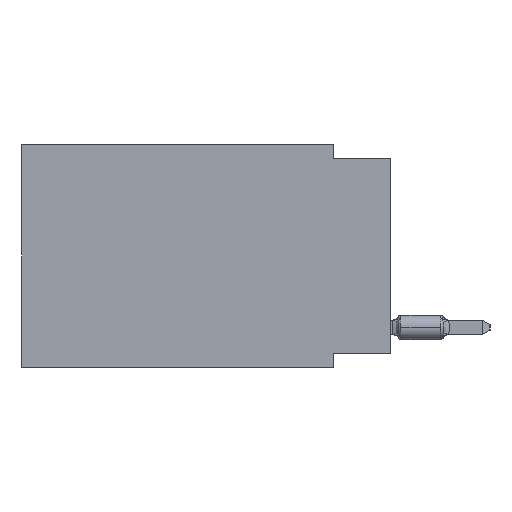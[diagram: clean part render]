
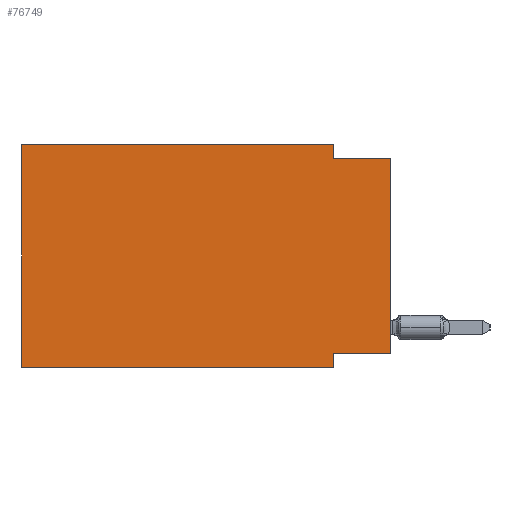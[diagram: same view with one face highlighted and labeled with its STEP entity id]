
A CAD part, left-side view. The second image highlights one B-rep face of the part: STEP entity #76749.
In plain terms, the highlighted planar face has unit normal (-1, 0, 0).
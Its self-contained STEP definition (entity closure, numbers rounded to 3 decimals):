
#1078 = CARTESIAN_POINT ( 'NONE',  ( 0., 0., -9.271 ) ) ;
#1573 = VECTOR ( 'NONE', #29314, 1000. ) ;
#2307 = EDGE_CURVE ( 'NONE', #81047, #10856, #3593, .T. ) ;
#3593 = LINE ( 'NONE', #55426, #55596 ) ;
#5826 = EDGE_CURVE ( 'NONE', #47652, #61496, #57460, .T. ) ;
#7304 = VECTOR ( 'NONE', #48601, 1000. ) ;
#8265 = EDGE_CURVE ( 'NONE', #61496, #81852, #83318, .T. ) ;
#9285 = CARTESIAN_POINT ( 'NONE',  ( 0., 2.54, -9.271 ) ) ;
#9320 = FACE_OUTER_BOUND ( 'NONE', #21078, .T. ) ;
#10399 = CARTESIAN_POINT ( 'NONE',  ( 0., 2.54, -9.906 ) ) ;
#10856 = VERTEX_POINT ( 'NONE', #16833 ) ;
#16367 = DIRECTION ( 'NONE',  ( 0., 0., -1. ) ) ;
#16833 = CARTESIAN_POINT ( 'NONE',  ( 0., 2.54, -9.906 ) ) ;
#18100 = ORIENTED_EDGE ( 'NONE', *, *, #40704, .F. ) ;
#21078 = EDGE_LOOP ( 'NONE', ( #23453, #83665, #46682, #51522, #18100, #27784, #24920, #65943 ) ) ;
#22477 = DIRECTION ( 'NONE',  ( 0., 0., -1. ) ) ;
#23117 = VERTEX_POINT ( 'NONE', #81016 ) ;
#23349 = CARTESIAN_POINT ( 'NONE',  ( 0., 0., 0. ) ) ;
#23400 = CARTESIAN_POINT ( 'NONE',  ( 0., 16.383, 0. ) ) ;
#23453 = ORIENTED_EDGE ( 'NONE', *, *, #25530, .T. ) ;
#24920 = ORIENTED_EDGE ( 'NONE', *, *, #61089, .F. ) ;
#25530 = EDGE_CURVE ( 'NONE', #64119, #81852, #73940, .T. ) ;
#27784 = ORIENTED_EDGE ( 'NONE', *, *, #2307, .T. ) ;
#28859 = CARTESIAN_POINT ( 'NONE',  ( 0., 16.383, 0. ) ) ;
#29314 = DIRECTION ( 'NONE',  ( 0., 0., 1. ) ) ;
#29662 = VECTOR ( 'NONE', #16367, 1000. ) ;
#30366 = LINE ( 'NONE', #10399, #29662 ) ;
#33137 = VECTOR ( 'NONE', #68941, 1000. ) ;
#35249 = PLANE ( 'NONE',  #65870 ) ;
#35443 = CARTESIAN_POINT ( 'NONE',  ( 0., 0., -9.271 ) ) ;
#36220 = EDGE_CURVE ( 'NONE', #64119, #68903, #67724, .T. ) ;
#37059 = CARTESIAN_POINT ( 'NONE',  ( 0., 16.383, -9.906 ) ) ;
#37674 = VECTOR ( 'NONE', #42556, 1000. ) ;
#40704 = EDGE_CURVE ( 'NONE', #81047, #23117, #56981, .T. ) ;
#42556 = DIRECTION ( 'NONE',  ( 0., 0., 1. ) ) ;
#43032 = CARTESIAN_POINT ( 'NONE',  ( 0., 2.54, 0. ) ) ;
#46682 = ORIENTED_EDGE ( 'NONE', *, *, #5826, .F. ) ;
#47134 = CARTESIAN_POINT ( 'NONE',  ( 0., 2.54, 0. ) ) ;
#47652 = VERTEX_POINT ( 'NONE', #47134 ) ;
#48601 = DIRECTION ( 'NONE',  ( 0., 1., 0. ) ) ;
#49036 = DIRECTION ( 'NONE',  ( 0., -1., 0. ) ) ;
#51522 = ORIENTED_EDGE ( 'NONE', *, *, #60721, .F. ) ;
#54775 = DIRECTION ( 'NONE',  ( 1., 0., 0. ) ) ;
#55426 = CARTESIAN_POINT ( 'NONE',  ( 0., 16.383, -9.906 ) ) ;
#55596 = VECTOR ( 'NONE', #49036, 1000. ) ;
#56981 = LINE ( 'NONE', #23400, #37674 ) ;
#57413 = DIRECTION ( 'NONE',  ( 0., -1., 0. ) ) ;
#57460 = LINE ( 'NONE', #43032, #33137 ) ;
#59535 = VECTOR ( 'NONE', #64476, 1000. ) ;
#60721 = EDGE_CURVE ( 'NONE', #23117, #47652, #70424, .T. ) ;
#61089 = EDGE_CURVE ( 'NONE', #68903, #10856, #30366, .T. ) ;
#61496 = VERTEX_POINT ( 'NONE', #68525 ) ;
#63786 = CARTESIAN_POINT ( 'NONE',  ( 0., 0., -0.635 ) ) ;
#64119 = VERTEX_POINT ( 'NONE', #1078 ) ;
#64476 = DIRECTION ( 'NONE',  ( 0., -1., 0. ) ) ;
#64488 = CARTESIAN_POINT ( 'NONE',  ( 0., 0., -0.635 ) ) ;
#65870 = AXIS2_PLACEMENT_3D ( 'NONE', #28859, #54775, #22477 ) ;
#65943 = ORIENTED_EDGE ( 'NONE', *, *, #36220, .F. ) ;
#67724 = LINE ( 'NONE', #35443, #7304 ) ;
#68525 = CARTESIAN_POINT ( 'NONE',  ( 0., 2.54, -0.635 ) ) ;
#68903 = VERTEX_POINT ( 'NONE', #9285 ) ;
#68941 = DIRECTION ( 'NONE',  ( 0., 0., -1. ) ) ;
#68954 = VECTOR ( 'NONE', #57413, 1000. ) ;
#70424 = LINE ( 'NONE', #84008, #59535 ) ;
#73940 = LINE ( 'NONE', #23349, #1573 ) ;
#76749 = ADVANCED_FACE ( 'NONE', ( #9320 ), #35249, .F. ) ;
#81016 = CARTESIAN_POINT ( 'NONE',  ( 0., 16.383, 0. ) ) ;
#81047 = VERTEX_POINT ( 'NONE', #37059 ) ;
#81852 = VERTEX_POINT ( 'NONE', #64488 ) ;
#83318 = LINE ( 'NONE', #63786, #68954 ) ;
#83665 = ORIENTED_EDGE ( 'NONE', *, *, #8265, .F. ) ;
#84008 = CARTESIAN_POINT ( 'NONE',  ( 0., 16.383, 0. ) ) ;
